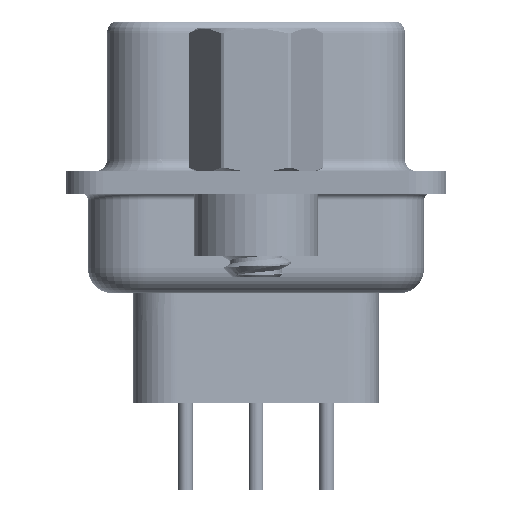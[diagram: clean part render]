
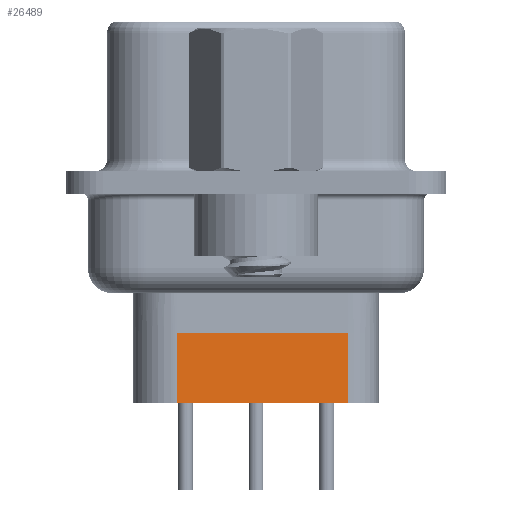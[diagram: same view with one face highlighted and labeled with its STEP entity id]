
A CAD part, left-side view. The second image highlights one B-rep face of the part: STEP entity #26489.
In plain terms, the highlighted planar face has unit normal (-0.985, -0.174, 0).
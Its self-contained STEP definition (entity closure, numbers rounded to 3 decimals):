
#123 = CARTESIAN_POINT ( 'NONE',  ( 4.574, 3.165, -6.05 ) ) ;
#355 = AXIS2_PLACEMENT_3D ( 'NONE', #38455, #21385, #17795 ) ;
#2151 = EDGE_LOOP ( 'NONE', ( #28602, #3115, #19733, #10797 ) ) ;
#3115 = ORIENTED_EDGE ( 'NONE', *, *, #16386, .T. ) ;
#4740 = EDGE_CURVE ( 'NONE', #37883, #41233, #26383, .T. ) ;
#5387 = VERTEX_POINT ( 'NONE', #22427 ) ;
#6296 = VECTOR ( 'NONE', #20649, 1000. ) ;
#6956 = LINE ( 'NONE', #41540, #6296 ) ;
#8340 = PLANE ( 'NONE',  #355 ) ;
#8525 = VECTOR ( 'NONE', #27892, 1000. ) ;
#10797 = ORIENTED_EDGE ( 'NONE', *, *, #19701, .F. ) ;
#14189 = LINE ( 'NONE', #27852, #43809 ) ;
#14884 = FACE_OUTER_BOUND ( 'NONE', #2151, .T. ) ;
#15204 = CARTESIAN_POINT ( 'NONE',  ( 4.574, 3.165, -3.1 ) ) ;
#16386 = EDGE_CURVE ( 'NONE', #5387, #37883, #18250, .T. ) ;
#16754 = CARTESIAN_POINT ( 'NONE',  ( 4.574, 3.165, -6.05 ) ) ;
#17795 = DIRECTION ( 'NONE',  ( 0.174, -0.985, 0. ) ) ;
#18054 = CARTESIAN_POINT ( 'NONE',  ( 4.574, 3.165, -8.85 ) ) ;
#18250 = LINE ( 'NONE', #16754, #8525 ) ;
#19701 = EDGE_CURVE ( 'NONE', #39575, #41233, #14189, .T. ) ;
#19733 = ORIENTED_EDGE ( 'NONE', *, *, #4740, .T. ) ;
#20649 = DIRECTION ( 'NONE',  ( 0., 0., -1. ) ) ;
#21385 = DIRECTION ( 'NONE',  ( -0.985, -0.174, 0. ) ) ;
#22427 = CARTESIAN_POINT ( 'NONE',  ( 5.781, -3.685, -6.05 ) ) ;
#24500 = DIRECTION ( 'NONE',  ( -0.174, 0.985, 0. ) ) ;
#25907 = CARTESIAN_POINT ( 'NONE',  ( 5.781, -3.685, -8.85 ) ) ;
#26383 = LINE ( 'NONE', #15204, #39511 ) ;
#26489 = ADVANCED_FACE ( 'NONE', ( #14884 ), #8340, .T. ) ;
#27852 = CARTESIAN_POINT ( 'NONE',  ( 4.574, 3.165, -8.85 ) ) ;
#27892 = DIRECTION ( 'NONE',  ( -0.174, 0.985, 0. ) ) ;
#28602 = ORIENTED_EDGE ( 'NONE', *, *, #36809, .F. ) ;
#36809 = EDGE_CURVE ( 'NONE', #5387, #39575, #6956, .T. ) ;
#37883 = VERTEX_POINT ( 'NONE', #123 ) ;
#38455 = CARTESIAN_POINT ( 'NONE',  ( 4.574, 3.165, -3.1 ) ) ;
#39511 = VECTOR ( 'NONE', #40123, 1000. ) ;
#39575 = VERTEX_POINT ( 'NONE', #25907 ) ;
#40123 = DIRECTION ( 'NONE',  ( 0., 0., -1. ) ) ;
#41233 = VERTEX_POINT ( 'NONE', #18054 ) ;
#41540 = CARTESIAN_POINT ( 'NONE',  ( 5.781, -3.685, -3.1 ) ) ;
#43809 = VECTOR ( 'NONE', #24500, 1000. ) ;
